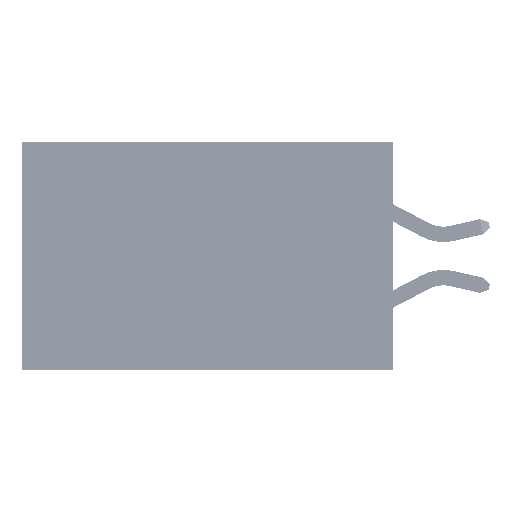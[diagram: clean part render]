
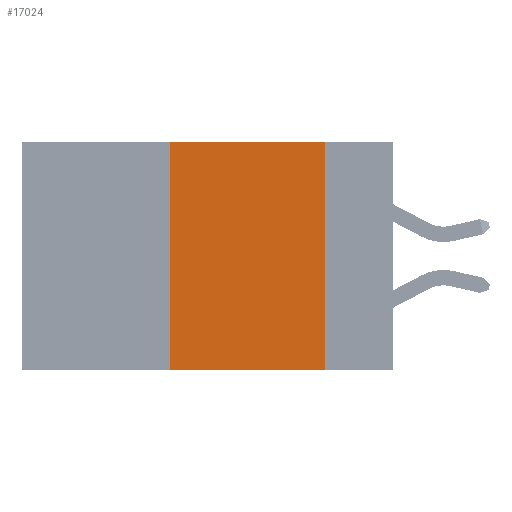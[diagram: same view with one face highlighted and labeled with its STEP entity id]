
A CAD part, left-side view. The second image highlights one B-rep face of the part: STEP entity #17024.
In plain terms, the highlighted planar face has unit normal (-1, 0, 0).
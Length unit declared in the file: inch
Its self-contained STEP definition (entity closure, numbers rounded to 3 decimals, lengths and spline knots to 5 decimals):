
#7122 = DIRECTION ( 'NONE',  ( 0., -1., 0. ) ) ;
#9039 = CARTESIAN_POINT ( 'NONE',  ( 0., 0.11, 0. ) ) ;
#9823 = ORIENTED_EDGE ( 'NONE', *, *, #26233, .T. ) ;
#10608 = CARTESIAN_POINT ( 'NONE',  ( 0., 0.36, 0. ) ) ;
#11219 = PLANE ( 'NONE',  #22826 ) ;
#11847 = VECTOR ( 'NONE', #43071, 39.37008 ) ;
#11917 = LINE ( 'NONE', #10608, #44608 ) ;
#14518 = VERTEX_POINT ( 'NONE', #31782 ) ;
#15101 = ORIENTED_EDGE ( 'NONE', *, *, #31469, .F. ) ;
#17024 = ADVANCED_FACE ( 'NONE', ( #47149 ), #11219, .F. ) ;
#17906 = ORIENTED_EDGE ( 'NONE', *, *, #39600, .F. ) ;
#19852 = VECTOR ( 'NONE', #7122, 39.37008 ) ;
#21704 = VERTEX_POINT ( 'NONE', #33309 ) ;
#22826 = AXIS2_PLACEMENT_3D ( 'NONE', #38800, #49752, #38306 ) ;
#22869 = EDGE_CURVE ( 'NONE', #29291, #21704, #11917, .T. ) ;
#23989 = CARTESIAN_POINT ( 'NONE',  ( 0., 0.11, 0. ) ) ;
#26233 = EDGE_CURVE ( 'NONE', #29291, #14518, #39734, .T. ) ;
#29291 = VERTEX_POINT ( 'NONE', #30228 ) ;
#30175 = LINE ( 'NONE', #30361, #19852 ) ;
#30228 = CARTESIAN_POINT ( 'NONE',  ( 0., 0.36, -0.37 ) ) ;
#30361 = CARTESIAN_POINT ( 'NONE',  ( 0., 0.6, 0. ) ) ;
#30815 = ORIENTED_EDGE ( 'NONE', *, *, #22869, .F. ) ;
#31469 = EDGE_CURVE ( 'NONE', #21704, #39715, #30175, .T. ) ;
#31782 = CARTESIAN_POINT ( 'NONE',  ( 0., 0.11, -0.37 ) ) ;
#32496 = LINE ( 'NONE', #23989, #41527 ) ;
#33309 = CARTESIAN_POINT ( 'NONE',  ( 0., 0.36, 0. ) ) ;
#35496 = CARTESIAN_POINT ( 'NONE',  ( 0., 0.6, -0.37 ) ) ;
#36414 = EDGE_LOOP ( 'NONE', ( #17906, #15101, #30815, #9823 ) ) ;
#37853 = DIRECTION ( 'NONE',  ( 0., 0., 1. ) ) ;
#38306 = DIRECTION ( 'NONE',  ( 0., 0., -1. ) ) ;
#38800 = CARTESIAN_POINT ( 'NONE',  ( 0., 0.6, 0. ) ) ;
#39600 = EDGE_CURVE ( 'NONE', #39715, #14518, #32496, .T. ) ;
#39715 = VERTEX_POINT ( 'NONE', #9039 ) ;
#39734 = LINE ( 'NONE', #35496, #11847 ) ;
#41527 = VECTOR ( 'NONE', #43207, 39.37008 ) ;
#43071 = DIRECTION ( 'NONE',  ( 0., -1., 0. ) ) ;
#43207 = DIRECTION ( 'NONE',  ( 0., 0., -1. ) ) ;
#44608 = VECTOR ( 'NONE', #37853, 39.37008 ) ;
#47149 = FACE_OUTER_BOUND ( 'NONE', #36414, .T. ) ;
#49752 = DIRECTION ( 'NONE',  ( 1., 0., 0. ) ) ;
